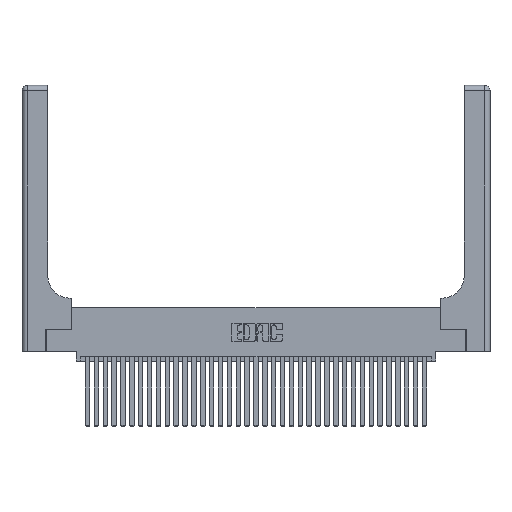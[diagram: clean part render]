
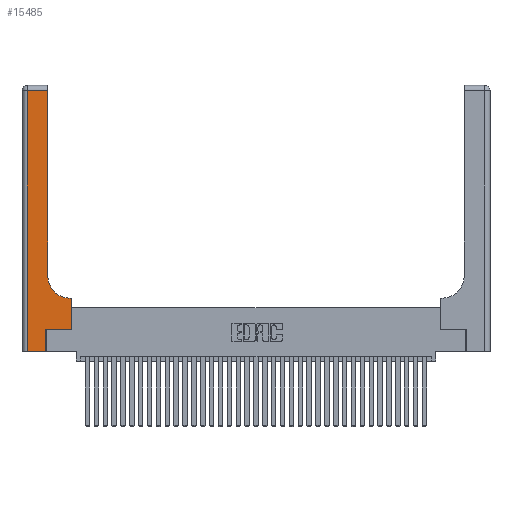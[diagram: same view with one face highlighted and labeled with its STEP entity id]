
A CAD part, top view. The second image highlights one B-rep face of the part: STEP entity #15485.
In plain terms, the highlighted planar face has unit normal (0, 0, 1).
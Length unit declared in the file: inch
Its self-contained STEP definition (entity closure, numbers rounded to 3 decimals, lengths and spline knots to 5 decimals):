
#646 = DIRECTION ( 'NONE',  ( -1., 0., 0. ) ) ;
#741 = CARTESIAN_POINT ( 'NONE',  ( 0.269, 0., 0.37 ) ) ;
#742 = CARTESIAN_POINT ( 'NONE',  ( 0.5415, 0.6, 0.37 ) ) ;
#1469 = VERTEX_POINT ( 'NONE', #22022 ) ;
#1789 = CARTESIAN_POINT ( 'NONE',  ( 0.269, 0.25, 0.37 ) ) ;
#3083 = CARTESIAN_POINT ( 'NONE',  ( 0.5415, 0.85, 0.37 ) ) ;
#4867 = ORIENTED_EDGE ( 'NONE', *, *, #9875, .T. ) ;
#5454 = VERTEX_POINT ( 'NONE', #742 ) ;
#5511 = CARTESIAN_POINT ( 'NONE',  ( 0.5585, 0.6, 0.37 ) ) ;
#5679 = ORIENTED_EDGE ( 'NONE', *, *, #22991, .T. ) ;
#5744 = CARTESIAN_POINT ( 'NONE',  ( 0.269, 0., 0.37 ) ) ;
#5794 = VECTOR ( 'NONE', #7444, 39.37008 ) ;
#5949 = DIRECTION ( 'NONE',  ( 1., 0., 0. ) ) ;
#5994 = LINE ( 'NONE', #25947, #34716 ) ;
#6413 = AXIS2_PLACEMENT_3D ( 'NONE', #34072, #17494, #646 ) ;
#6664 = VERTEX_POINT ( 'NONE', #5744 ) ;
#6972 = DIRECTION ( 'NONE',  ( 1., 0., 0. ) ) ;
#6987 = ORIENTED_EDGE ( 'NONE', *, *, #30881, .T. ) ;
#7444 = DIRECTION ( 'NONE',  ( 1., 0., 0. ) ) ;
#7453 = ORIENTED_EDGE ( 'NONE', *, *, #11983, .T. ) ;
#7888 = VERTEX_POINT ( 'NONE', #19391 ) ;
#8401 = FACE_OUTER_BOUND ( 'NONE', #22495, .T. ) ;
#8446 = EDGE_CURVE ( 'NONE', #7888, #24467, #34994, .T. ) ;
#9126 = ORIENTED_EDGE ( 'NONE', *, *, #16068, .T. ) ;
#9144 = DIRECTION ( 'NONE',  ( 0., 1., 0. ) ) ;
#9350 = CARTESIAN_POINT ( 'NONE',  ( 0.06, 0., 0.37 ) ) ;
#9358 = CARTESIAN_POINT ( 'NONE',  ( 0.269, 0.25, 0.37 ) ) ;
#9402 = DIRECTION ( 'NONE',  ( 0., 1., 0. ) ) ;
#9796 = CARTESIAN_POINT ( 'NONE',  ( 0., 0., 0.37 ) ) ;
#9875 = EDGE_CURVE ( 'NONE', #6664, #35249, #16257, .T. ) ;
#10474 = VERTEX_POINT ( 'NONE', #9350 ) ;
#11629 = LINE ( 'NONE', #23099, #18214 ) ;
#11866 = PLANE ( 'NONE',  #6413 ) ;
#11983 = EDGE_CURVE ( 'NONE', #1469, #7888, #5994, .T. ) ;
#12871 = VECTOR ( 'NONE', #20005, 39.37008 ) ;
#13260 = LINE ( 'NONE', #26981, #19835 ) ;
#13606 = ORIENTED_EDGE ( 'NONE', *, *, #30847, .T. ) ;
#14294 = ORIENTED_EDGE ( 'NONE', *, *, #25109, .T. ) ;
#15485 = ADVANCED_FACE ( 'NONE', ( #8401 ), #11866, .F. ) ;
#15745 = VECTOR ( 'NONE', #6972, 39.37008 ) ;
#15984 = ORIENTED_EDGE ( 'NONE', *, *, #8446, .T. ) ;
#16068 = EDGE_CURVE ( 'NONE', #5454, #1469, #18896, .T. ) ;
#16187 = VERTEX_POINT ( 'NONE', #23223 ) ;
#16257 = LINE ( 'NONE', #741, #29283 ) ;
#17494 = DIRECTION ( 'NONE',  ( 0., 0., -1. ) ) ;
#17821 = DIRECTION ( 'NONE',  ( 0., -1., 0. ) ) ;
#18158 = VERTEX_POINT ( 'NONE', #5511 ) ;
#18214 = VECTOR ( 'NONE', #9144, 39.37008 ) ;
#18740 = DIRECTION ( 'NONE',  ( -1., 0., 0. ) ) ;
#18896 = CIRCLE ( 'NONE', #26310, 0.25 ) ;
#19391 = CARTESIAN_POINT ( 'NONE',  ( 0.2915, 2.94, 0.37 ) ) ;
#19835 = VECTOR ( 'NONE', #18740, 39.37008 ) ;
#20005 = DIRECTION ( 'NONE',  ( -1., 0., 0. ) ) ;
#20411 = ORIENTED_EDGE ( 'NONE', *, *, #21659, .T. ) ;
#21659 = EDGE_CURVE ( 'NONE', #24467, #10474, #28869, .T. ) ;
#22022 = CARTESIAN_POINT ( 'NONE',  ( 0.2915, 0.85, 0.37 ) ) ;
#22495 = EDGE_LOOP ( 'NONE', ( #7453, #15984, #20411, #5679, #4867, #13606, #14294, #6987, #9126 ) ) ;
#22745 = DIRECTION ( 'NONE',  ( 0., 0., -1. ) ) ;
#22991 = EDGE_CURVE ( 'NONE', #10474, #6664, #24055, .T. ) ;
#23099 = CARTESIAN_POINT ( 'NONE',  ( 0.5585, 0.25, 0.37 ) ) ;
#23223 = CARTESIAN_POINT ( 'NONE',  ( 0.5585, 0.25, 0.37 ) ) ;
#24055 = LINE ( 'NONE', #9796, #15745 ) ;
#24467 = VERTEX_POINT ( 'NONE', #28289 ) ;
#25109 = EDGE_CURVE ( 'NONE', #16187, #18158, #11629, .T. ) ;
#25947 = CARTESIAN_POINT ( 'NONE',  ( 0.2915, 3., 0.37 ) ) ;
#26310 = AXIS2_PLACEMENT_3D ( 'NONE', #3083, #22745, #5949 ) ;
#26981 = CARTESIAN_POINT ( 'NONE',  ( 0.2915, 0.6, 0.37 ) ) ;
#27138 = VECTOR ( 'NONE', #17821, 39.37008 ) ;
#28051 = LINE ( 'NONE', #1789, #5794 ) ;
#28289 = CARTESIAN_POINT ( 'NONE',  ( 0.06, 2.94, 0.37 ) ) ;
#28708 = DIRECTION ( 'NONE',  ( 0., 1., 0. ) ) ;
#28869 = LINE ( 'NONE', #31606, #27138 ) ;
#29283 = VECTOR ( 'NONE', #9402, 39.37008 ) ;
#30847 = EDGE_CURVE ( 'NONE', #35249, #16187, #28051, .T. ) ;
#30881 = EDGE_CURVE ( 'NONE', #18158, #5454, #13260, .T. ) ;
#30976 = CARTESIAN_POINT ( 'NONE',  ( 0., 2.94, 0.37 ) ) ;
#31606 = CARTESIAN_POINT ( 'NONE',  ( 0.06, 3., 0.37 ) ) ;
#34072 = CARTESIAN_POINT ( 'NONE',  ( 0., 3., 0.37 ) ) ;
#34716 = VECTOR ( 'NONE', #28708, 39.37008 ) ;
#34994 = LINE ( 'NONE', #30976, #12871 ) ;
#35249 = VERTEX_POINT ( 'NONE', #9358 ) ;
